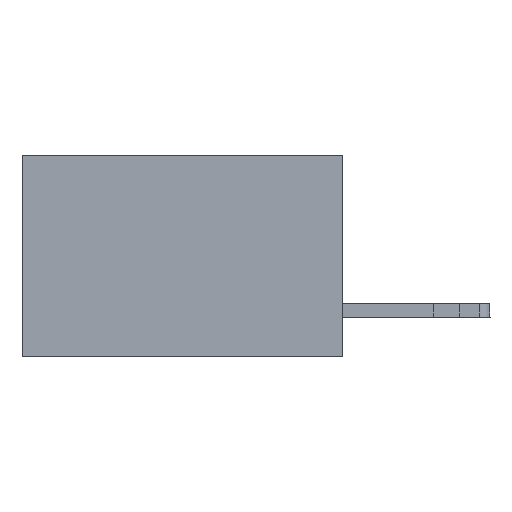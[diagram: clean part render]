
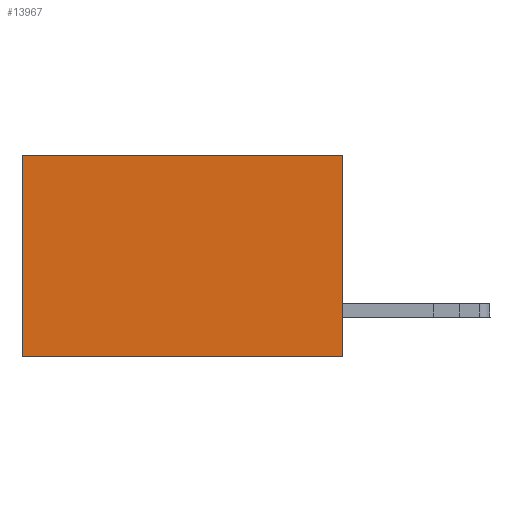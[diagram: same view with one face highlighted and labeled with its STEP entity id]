
A CAD part, left-side view. The second image highlights one B-rep face of the part: STEP entity #13967.
In plain terms, the highlighted planar face has unit normal (-1, 0, 0).
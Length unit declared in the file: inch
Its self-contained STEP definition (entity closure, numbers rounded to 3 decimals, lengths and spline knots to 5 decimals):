
#2212 = VECTOR ( 'NONE', #15818, 39.37008 ) ;
#2327 = EDGE_LOOP ( 'NONE', ( #8735, #9280, #24612, #22355 ) ) ;
#2695 = EDGE_CURVE ( 'NONE', #14637, #29839, #28277, .T. ) ;
#2840 = VERTEX_POINT ( 'NONE', #29110 ) ;
#3727 = CARTESIAN_POINT ( 'NONE',  ( 0.277, 0., -0.37 ) ) ;
#5805 = CARTESIAN_POINT ( 'NONE',  ( 0.277, 0., -0.37 ) ) ;
#6300 = PLANE ( 'NONE',  #11815 ) ;
#6423 = CARTESIAN_POINT ( 'NONE',  ( 0.277, 0.59, 0. ) ) ;
#6756 = CARTESIAN_POINT ( 'NONE',  ( 0.277, 0., 0. ) ) ;
#7337 = VECTOR ( 'NONE', #28698, 39.37008 ) ;
#8735 = ORIENTED_EDGE ( 'NONE', *, *, #31479, .T. ) ;
#8841 = CARTESIAN_POINT ( 'NONE',  ( 0.277, 0.59, -0.37 ) ) ;
#9280 = ORIENTED_EDGE ( 'NONE', *, *, #31962, .F. ) ;
#9891 = LINE ( 'NONE', #26989, #23052 ) ;
#11815 = AXIS2_PLACEMENT_3D ( 'NONE', #5805, #16144, #26152 ) ;
#13374 = CARTESIAN_POINT ( 'NONE',  ( 0.277, 0., 0. ) ) ;
#13967 = ADVANCED_FACE ( 'NONE', ( #28280 ), #6300, .F. ) ;
#14637 = VERTEX_POINT ( 'NONE', #6756 ) ;
#15818 = DIRECTION ( 'NONE',  ( 0., 1., 0. ) ) ;
#16144 = DIRECTION ( 'NONE',  ( 1., 0., 0. ) ) ;
#17210 = EDGE_CURVE ( 'NONE', #14637, #19289, #26210, .T. ) ;
#18681 = LINE ( 'NONE', #8841, #7337 ) ;
#19289 = VERTEX_POINT ( 'NONE', #22380 ) ;
#19426 = DIRECTION ( 'NONE',  ( 0., 1., 0. ) ) ;
#21512 = VECTOR ( 'NONE', #28673, 39.37008 ) ;
#22355 = ORIENTED_EDGE ( 'NONE', *, *, #2695, .T. ) ;
#22380 = CARTESIAN_POINT ( 'NONE',  ( 0.277, 0., -0.37 ) ) ;
#23052 = VECTOR ( 'NONE', #19426, 39.37008 ) ;
#24612 = ORIENTED_EDGE ( 'NONE', *, *, #17210, .F. ) ;
#26152 = DIRECTION ( 'NONE',  ( 0., 0., -1. ) ) ;
#26210 = LINE ( 'NONE', #3727, #21512 ) ;
#26989 = CARTESIAN_POINT ( 'NONE',  ( 0.277, 0., -0.37 ) ) ;
#28277 = LINE ( 'NONE', #13374, #2212 ) ;
#28280 = FACE_OUTER_BOUND ( 'NONE', #2327, .T. ) ;
#28673 = DIRECTION ( 'NONE',  ( 0., 0., -1. ) ) ;
#28698 = DIRECTION ( 'NONE',  ( 0., 0., -1. ) ) ;
#29110 = CARTESIAN_POINT ( 'NONE',  ( 0.277, 0.59, -0.37 ) ) ;
#29839 = VERTEX_POINT ( 'NONE', #6423 ) ;
#31479 = EDGE_CURVE ( 'NONE', #29839, #2840, #18681, .T. ) ;
#31962 = EDGE_CURVE ( 'NONE', #19289, #2840, #9891, .T. ) ;
